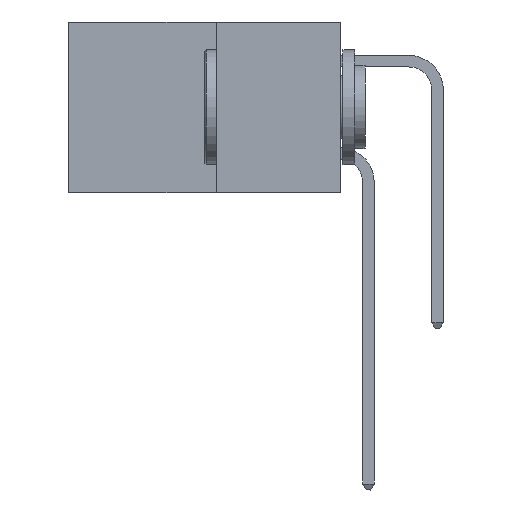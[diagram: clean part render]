
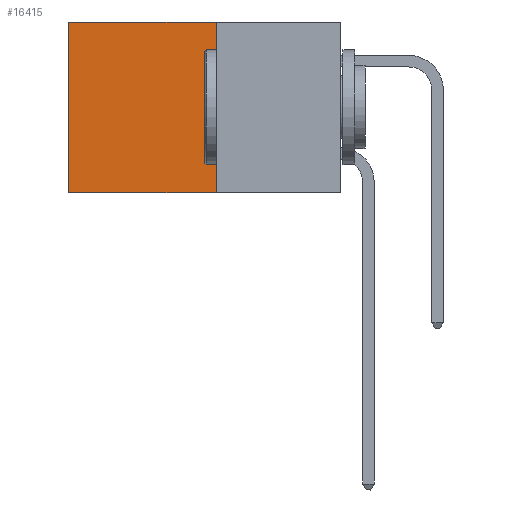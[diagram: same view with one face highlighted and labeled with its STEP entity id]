
A CAD part, left-side view. The second image highlights one B-rep face of the part: STEP entity #16415.
In plain terms, the highlighted planar face has unit normal (-1, 0, 0).
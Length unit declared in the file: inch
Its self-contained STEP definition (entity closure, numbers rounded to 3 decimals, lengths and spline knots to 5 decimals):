
#556 = ORIENTED_EDGE ( 'NONE', *, *, #14925, .F. ) ;
#1382 = LINE ( 'NONE', #10098, #9427 ) ;
#1630 = EDGE_CURVE ( 'NONE', #12111, #18410, #16390, .T. ) ;
#1718 = DIRECTION ( 'NONE',  ( 0., 1., 0. ) ) ;
#2158 = PLANE ( 'NONE',  #5975 ) ;
#2491 = ORIENTED_EDGE ( 'NONE', *, *, #1630, .F. ) ;
#3716 = VECTOR ( 'NONE', #1718, 39.37008 ) ;
#3850 = CARTESIAN_POINT ( 'NONE',  ( 0.277, 0.27, -0.37 ) ) ;
#4128 = CARTESIAN_POINT ( 'NONE',  ( 0.277, 0.27, -0.37 ) ) ;
#4704 = CARTESIAN_POINT ( 'NONE',  ( 0.277, 0.27, -0.37 ) ) ;
#5494 = DIRECTION ( 'NONE',  ( 1., 0., 0. ) ) ;
#5975 = AXIS2_PLACEMENT_3D ( 'NONE', #3850, #5494, #16549 ) ;
#6469 = VERTEX_POINT ( 'NONE', #9188 ) ;
#6836 = FACE_OUTER_BOUND ( 'NONE', #10665, .T. ) ;
#7333 = LINE ( 'NONE', #17064, #17951 ) ;
#8398 = EDGE_CURVE ( 'NONE', #15738, #6469, #7333, .T. ) ;
#8616 = CARTESIAN_POINT ( 'NONE',  ( 0.277, 0.27, -0.37 ) ) ;
#8789 = CARTESIAN_POINT ( 'NONE',  ( 0.277, 0.59, -0.37 ) ) ;
#9188 = CARTESIAN_POINT ( 'NONE',  ( 0.277, 0.59, 0. ) ) ;
#9269 = CARTESIAN_POINT ( 'NONE',  ( 0.277, 0.27, 0. ) ) ;
#9427 = VECTOR ( 'NONE', #11679, 39.37008 ) ;
#10098 = CARTESIAN_POINT ( 'NONE',  ( 0.277, 0.59, -0.37 ) ) ;
#10458 = EDGE_CURVE ( 'NONE', #6469, #18410, #1382, .T. ) ;
#10665 = EDGE_LOOP ( 'NONE', ( #16307, #2491, #556, #16676 ) ) ;
#11679 = DIRECTION ( 'NONE',  ( 0., 0., -1. ) ) ;
#11935 = DIRECTION ( 'NONE',  ( 0., 0., -1. ) ) ;
#12111 = VERTEX_POINT ( 'NONE', #4704 ) ;
#14925 = EDGE_CURVE ( 'NONE', #15738, #12111, #16266, .T. ) ;
#15738 = VERTEX_POINT ( 'NONE', #9269 ) ;
#16266 = LINE ( 'NONE', #4128, #20363 ) ;
#16307 = ORIENTED_EDGE ( 'NONE', *, *, #10458, .T. ) ;
#16390 = LINE ( 'NONE', #8616, #3716 ) ;
#16415 = ADVANCED_FACE ( 'NONE', ( #6836 ), #2158, .F. ) ;
#16549 = DIRECTION ( 'NONE',  ( 0., 0., -1. ) ) ;
#16676 = ORIENTED_EDGE ( 'NONE', *, *, #8398, .T. ) ;
#16845 = DIRECTION ( 'NONE',  ( 0., 1., 0. ) ) ;
#17064 = CARTESIAN_POINT ( 'NONE',  ( 0.277, 0.27, 0. ) ) ;
#17951 = VECTOR ( 'NONE', #16845, 39.37008 ) ;
#18410 = VERTEX_POINT ( 'NONE', #8789 ) ;
#20363 = VECTOR ( 'NONE', #11935, 39.37008 ) ;
